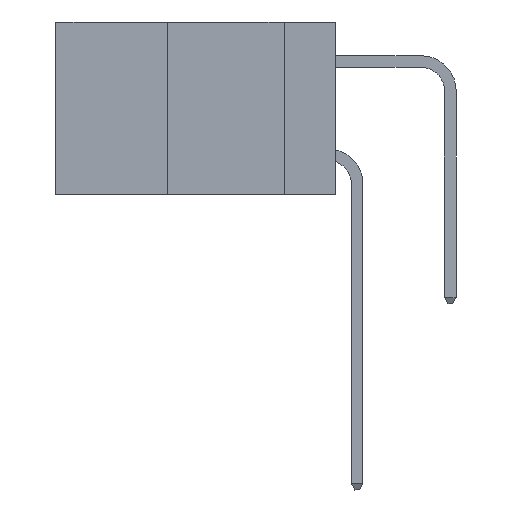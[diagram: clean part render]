
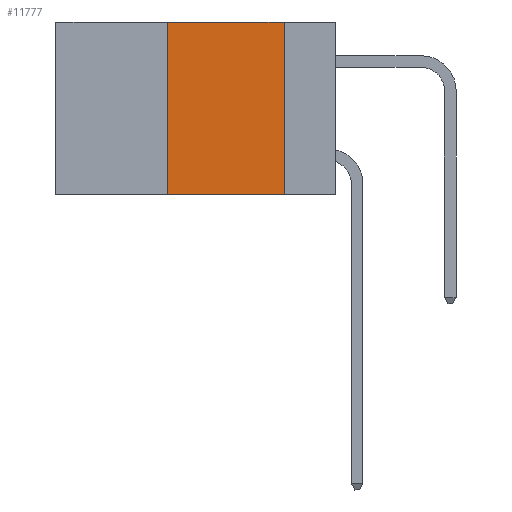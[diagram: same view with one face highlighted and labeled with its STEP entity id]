
A CAD part, left-side view. The second image highlights one B-rep face of the part: STEP entity #11777.
In plain terms, the highlighted planar face has unit normal (-1, 0, 0).
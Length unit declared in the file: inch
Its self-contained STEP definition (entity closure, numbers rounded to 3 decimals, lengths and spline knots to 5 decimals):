
#1613 = DIRECTION ( 'NONE',  ( 0., 0., -1. ) ) ;
#2288 = DIRECTION ( 'NONE',  ( 0., -1., 0. ) ) ;
#2572 = CARTESIAN_POINT ( 'NONE',  ( 0., 0.6, -0.37 ) ) ;
#3010 = AXIS2_PLACEMENT_3D ( 'NONE', #8072, #17426, #1613 ) ;
#3340 = ORIENTED_EDGE ( 'NONE', *, *, #3786, .F. ) ;
#3786 = EDGE_CURVE ( 'NONE', #16023, #19442, #4126, .T. ) ;
#4097 = CARTESIAN_POINT ( 'NONE',  ( 0., 0.6, 0. ) ) ;
#4126 = LINE ( 'NONE', #5590, #10004 ) ;
#4996 = CARTESIAN_POINT ( 'NONE',  ( 0., 0.36, 0. ) ) ;
#5590 = CARTESIAN_POINT ( 'NONE',  ( 0., 0.11, 0. ) ) ;
#6448 = VECTOR ( 'NONE', #18623, 39.37008 ) ;
#7965 = EDGE_CURVE ( 'NONE', #10468, #13528, #15929, .T. ) ;
#8072 = CARTESIAN_POINT ( 'NONE',  ( 0., 0.6, 0. ) ) ;
#9032 = ORIENTED_EDGE ( 'NONE', *, *, #7965, .F. ) ;
#10004 = VECTOR ( 'NONE', #11520, 39.37008 ) ;
#10468 = VERTEX_POINT ( 'NONE', #11356 ) ;
#11356 = CARTESIAN_POINT ( 'NONE',  ( 0., 0.36, -0.37 ) ) ;
#11520 = DIRECTION ( 'NONE',  ( 0., 0., -1. ) ) ;
#11777 = ADVANCED_FACE ( 'NONE', ( #19416 ), #18496, .F. ) ;
#12440 = DIRECTION ( 'NONE',  ( 0., 0., 1. ) ) ;
#13528 = VERTEX_POINT ( 'NONE', #4996 ) ;
#13761 = VECTOR ( 'NONE', #2288, 39.37008 ) ;
#14701 = CARTESIAN_POINT ( 'NONE',  ( 0., 0.11, -0.37 ) ) ;
#14802 = CARTESIAN_POINT ( 'NONE',  ( 0., 0.11, 0. ) ) ;
#15455 = EDGE_CURVE ( 'NONE', #13528, #16023, #15703, .T. ) ;
#15615 = EDGE_LOOP ( 'NONE', ( #3340, #19670, #9032, #15900 ) ) ;
#15703 = LINE ( 'NONE', #4097, #13761 ) ;
#15899 = LINE ( 'NONE', #2572, #6448 ) ;
#15900 = ORIENTED_EDGE ( 'NONE', *, *, #17322, .T. ) ;
#15929 = LINE ( 'NONE', #22862, #20035 ) ;
#16023 = VERTEX_POINT ( 'NONE', #14802 ) ;
#17322 = EDGE_CURVE ( 'NONE', #10468, #19442, #15899, .T. ) ;
#17426 = DIRECTION ( 'NONE',  ( 1., 0., 0. ) ) ;
#18496 = PLANE ( 'NONE',  #3010 ) ;
#18623 = DIRECTION ( 'NONE',  ( 0., -1., 0. ) ) ;
#19416 = FACE_OUTER_BOUND ( 'NONE', #15615, .T. ) ;
#19442 = VERTEX_POINT ( 'NONE', #14701 ) ;
#19670 = ORIENTED_EDGE ( 'NONE', *, *, #15455, .F. ) ;
#20035 = VECTOR ( 'NONE', #12440, 39.37008 ) ;
#22862 = CARTESIAN_POINT ( 'NONE',  ( 0., 0.36, 0. ) ) ;
